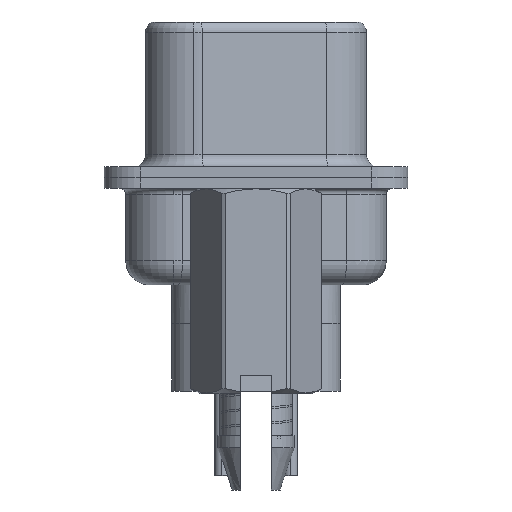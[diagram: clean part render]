
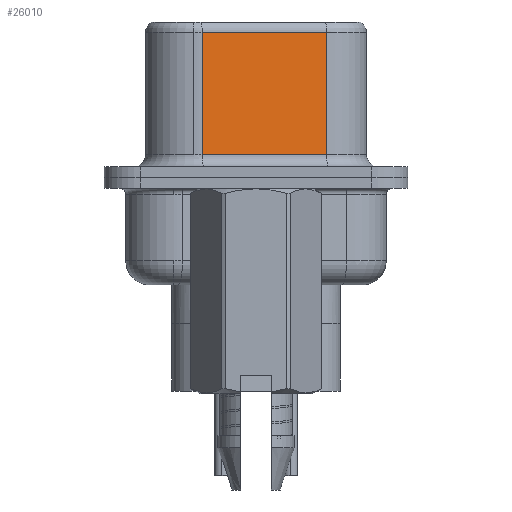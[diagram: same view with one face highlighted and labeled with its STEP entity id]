
A CAD part, left-side view. The second image highlights one B-rep face of the part: STEP entity #26010.
In plain terms, the highlighted planar face has unit normal (-0.985, -0.174, 0).
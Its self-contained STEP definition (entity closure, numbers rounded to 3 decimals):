
#634 = VERTEX_POINT ( 'NONE', #19062 ) ;
#691 = VECTOR ( 'NONE', #26389, 1000. ) ;
#1062 = FACE_OUTER_BOUND ( 'NONE', #22052, .T. ) ;
#1256 = VERTEX_POINT ( 'NONE', #7590 ) ;
#1268 = CARTESIAN_POINT ( 'NONE',  ( 4.575, -2.927, 6.52 ) ) ;
#4497 = DIRECTION ( 'NONE',  ( -0.174, 0.985, 0. ) ) ;
#4828 = ORIENTED_EDGE ( 'NONE', *, *, #15430, .F. ) ;
#5330 = EDGE_CURVE ( 'NONE', #1256, #23601, #23402, .T. ) ;
#7462 = CARTESIAN_POINT ( 'NONE',  ( 4.575, -2.927, 6.02 ) ) ;
#7590 = CARTESIAN_POINT ( 'NONE',  ( 4.575, -2.927, 6.02 ) ) ;
#7646 = ORIENTED_EDGE ( 'NONE', *, *, #5330, .T. ) ;
#7930 = CARTESIAN_POINT ( 'NONE',  ( 4.575, -2.927, 6.52 ) ) ;
#10647 = CARTESIAN_POINT ( 'NONE',  ( 3.665, 2.233, 6.52 ) ) ;
#12943 = VECTOR ( 'NONE', #20102, 1000. ) ;
#13251 = LINE ( 'NONE', #28210, #19992 ) ;
#15430 = EDGE_CURVE ( 'NONE', #1256, #35033, #20679, .T. ) ;
#15861 = DIRECTION ( 'NONE',  ( 0.985, 0.174, 0. ) ) ;
#16615 = EDGE_CURVE ( 'NONE', #634, #35033, #13251, .T. ) ;
#19062 = CARTESIAN_POINT ( 'NONE',  ( 3.665, 2.233, 0.95 ) ) ;
#19992 = VECTOR ( 'NONE', #37405, 1000. ) ;
#20102 = DIRECTION ( 'NONE',  ( 0., 0., -1. ) ) ;
#20679 = LINE ( 'NONE', #7930, #12943 ) ;
#22052 = EDGE_LOOP ( 'NONE', ( #4828, #7646, #37031, #24557 ) ) ;
#23402 = LINE ( 'NONE', #7462, #30460 ) ;
#23601 = VERTEX_POINT ( 'NONE', #37159 ) ;
#24557 = ORIENTED_EDGE ( 'NONE', *, *, #16615, .T. ) ;
#25022 = PLANE ( 'NONE',  #36708 ) ;
#26010 = ADVANCED_FACE ( 'NONE', ( #1062 ), #25022, .F. ) ;
#26389 = DIRECTION ( 'NONE',  ( 0., 0., -1. ) ) ;
#28210 = CARTESIAN_POINT ( 'NONE',  ( 4.575, -2.927, 0.95 ) ) ;
#30460 = VECTOR ( 'NONE', #4497, 1000. ) ;
#31598 = LINE ( 'NONE', #10647, #691 ) ;
#35033 = VERTEX_POINT ( 'NONE', #38616 ) ;
#35678 = EDGE_CURVE ( 'NONE', #23601, #634, #31598, .T. ) ;
#36708 = AXIS2_PLACEMENT_3D ( 'NONE', #1268, #15861, #37214 ) ;
#37031 = ORIENTED_EDGE ( 'NONE', *, *, #35678, .T. ) ;
#37159 = CARTESIAN_POINT ( 'NONE',  ( 3.665, 2.233, 6.02 ) ) ;
#37214 = DIRECTION ( 'NONE',  ( -0.174, 0.985, 0. ) ) ;
#37405 = DIRECTION ( 'NONE',  ( 0.174, -0.985, 0. ) ) ;
#38616 = CARTESIAN_POINT ( 'NONE',  ( 4.575, -2.927, 0.95 ) ) ;
